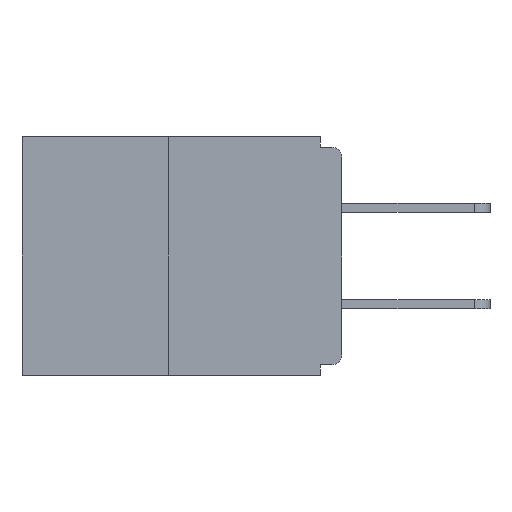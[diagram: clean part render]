
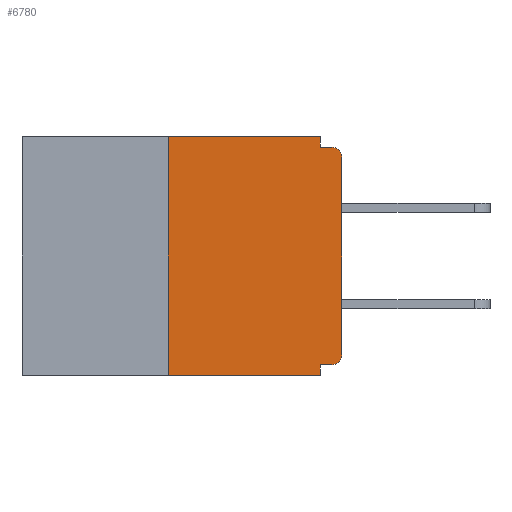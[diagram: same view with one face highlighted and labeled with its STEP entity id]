
A CAD part, left-side view. The second image highlights one B-rep face of the part: STEP entity #6780.
In plain terms, the highlighted planar face has unit normal (-1, 0, 0).
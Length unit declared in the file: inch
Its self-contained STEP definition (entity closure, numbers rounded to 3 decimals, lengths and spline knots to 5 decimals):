
#66 = CARTESIAN_POINT ( 'NONE',  ( 0., 0.031, 0. ) ) ;
#128 = CARTESIAN_POINT ( 'NONE',  ( 0., 0.015, -0.313 ) ) ;
#251 = CARTESIAN_POINT ( 'NONE',  ( 0., 0.031, -0.343 ) ) ;
#483 = DIRECTION ( 'NONE',  ( 1., 0., 0. ) ) ;
#576 = EDGE_CURVE ( 'NONE', #8437, #6505, #1379, .T. ) ;
#1377 = DIRECTION ( 'NONE',  ( 0., 0., -1. ) ) ;
#1379 = LINE ( 'NONE', #251, #6125 ) ;
#1640 = EDGE_CURVE ( 'NONE', #14112, #19363, #13053, .T. ) ;
#1816 = VERTEX_POINT ( 'NONE', #15189 ) ;
#2113 = LINE ( 'NONE', #4300, #10301 ) ;
#2531 = VECTOR ( 'NONE', #5734, 39.37008 ) ;
#2602 = FACE_OUTER_BOUND ( 'NONE', #16657, .T. ) ;
#3132 = EDGE_CURVE ( 'NONE', #1816, #14112, #12727, .T. ) ;
#3435 = CARTESIAN_POINT ( 'NONE',  ( 0., 0.031, 0. ) ) ;
#3496 = EDGE_CURVE ( 'NONE', #18222, #20248, #6762, .T. ) ;
#3988 = LINE ( 'NONE', #7442, #7696 ) ;
#4300 = CARTESIAN_POINT ( 'NONE',  ( 0., 0.46, -0.343 ) ) ;
#4327 = ORIENTED_EDGE ( 'NONE', *, *, #1640, .F. ) ;
#4531 = CARTESIAN_POINT ( 'NONE',  ( 0., 0.015, -0.015 ) ) ;
#4659 = DIRECTION ( 'NONE',  ( 0., 0., -1. ) ) ;
#5332 = CARTESIAN_POINT ( 'NONE',  ( 0., 0.031, -0.343 ) ) ;
#5734 = DIRECTION ( 'NONE',  ( 0., 0., 1. ) ) ;
#5997 = LINE ( 'NONE', #16172, #16929 ) ;
#6125 = VECTOR ( 'NONE', #15954, 39.37008 ) ;
#6214 = EDGE_CURVE ( 'NONE', #14409, #9686, #9053, .T. ) ;
#6505 = VERTEX_POINT ( 'NONE', #5332 ) ;
#6665 = CARTESIAN_POINT ( 'NONE',  ( 0., 0.46, 0. ) ) ;
#6762 = CIRCLE ( 'NONE', #8613, 0.015 ) ;
#6780 = ADVANCED_FACE ( 'NONE', ( #2602 ), #19461, .F. ) ;
#7053 = AXIS2_PLACEMENT_3D ( 'NONE', #6665, #483, #16252 ) ;
#7214 = EDGE_CURVE ( 'NONE', #12928, #6505, #2113, .T. ) ;
#7398 = DIRECTION ( 'NONE',  ( 0., 0., -1. ) ) ;
#7442 = CARTESIAN_POINT ( 'NONE',  ( 0., 0.25, 0. ) ) ;
#7696 = VECTOR ( 'NONE', #13715, 39.37008 ) ;
#8270 = DIRECTION ( 'NONE',  ( 0., 1., 0. ) ) ;
#8437 = VERTEX_POINT ( 'NONE', #9272 ) ;
#8613 = AXIS2_PLACEMENT_3D ( 'NONE', #9449, #10916, #1377 ) ;
#8761 = EDGE_CURVE ( 'NONE', #9686, #18222, #14700, .T. ) ;
#8899 = VECTOR ( 'NONE', #19779, 39.37008 ) ;
#9053 = CIRCLE ( 'NONE', #14910, 0.015 ) ;
#9259 = EDGE_CURVE ( 'NONE', #12928, #1816, #3988, .T. ) ;
#9272 = CARTESIAN_POINT ( 'NONE',  ( 0., 0.031, -0.328 ) ) ;
#9413 = ORIENTED_EDGE ( 'NONE', *, *, #8761, .T. ) ;
#9449 = CARTESIAN_POINT ( 'NONE',  ( 0., 0.015, -0.03 ) ) ;
#9601 = ORIENTED_EDGE ( 'NONE', *, *, #10444, .F. ) ;
#9686 = VERTEX_POINT ( 'NONE', #18036 ) ;
#10301 = VECTOR ( 'NONE', #10809, 39.37008 ) ;
#10444 = EDGE_CURVE ( 'NONE', #19363, #20248, #12618, .T. ) ;
#10809 = DIRECTION ( 'NONE',  ( 0., -1., 0. ) ) ;
#10916 = DIRECTION ( 'NONE',  ( -1., 0., 0. ) ) ;
#11150 = CARTESIAN_POINT ( 'NONE',  ( 0., 0.46, 0. ) ) ;
#11790 = ORIENTED_EDGE ( 'NONE', *, *, #19508, .F. ) ;
#12618 = LINE ( 'NONE', #18275, #8899 ) ;
#12727 = LINE ( 'NONE', #11150, #13249 ) ;
#12928 = VERTEX_POINT ( 'NONE', #14136 ) ;
#13053 = LINE ( 'NONE', #66, #14061 ) ;
#13249 = VECTOR ( 'NONE', #19274, 39.37008 ) ;
#13715 = DIRECTION ( 'NONE',  ( 0., 0., 1. ) ) ;
#14061 = VECTOR ( 'NONE', #4659, 39.37008 ) ;
#14112 = VERTEX_POINT ( 'NONE', #3435 ) ;
#14136 = CARTESIAN_POINT ( 'NONE',  ( 0., 0.25, -0.343 ) ) ;
#14409 = VERTEX_POINT ( 'NONE', #18959 ) ;
#14455 = DIRECTION ( 'NONE',  ( -1., 0., 0. ) ) ;
#14700 = LINE ( 'NONE', #15370, #2531 ) ;
#14910 = AXIS2_PLACEMENT_3D ( 'NONE', #128, #14455, #7398 ) ;
#15189 = CARTESIAN_POINT ( 'NONE',  ( 0., 0.25, 0. ) ) ;
#15370 = CARTESIAN_POINT ( 'NONE',  ( 0., 0., 0. ) ) ;
#15902 = CARTESIAN_POINT ( 'NONE',  ( 0., 0., -0.03 ) ) ;
#15954 = DIRECTION ( 'NONE',  ( 0., 0., -1. ) ) ;
#16172 = CARTESIAN_POINT ( 'NONE',  ( 0., 0., -0.328 ) ) ;
#16252 = DIRECTION ( 'NONE',  ( 0., 0., -1. ) ) ;
#16657 = EDGE_LOOP ( 'NONE', ( #17831, #20264, #17310, #20112, #11790, #16899, #9413, #17422, #9601, #4327 ) ) ;
#16899 = ORIENTED_EDGE ( 'NONE', *, *, #6214, .T. ) ;
#16929 = VECTOR ( 'NONE', #8270, 39.37008 ) ;
#17310 = ORIENTED_EDGE ( 'NONE', *, *, #7214, .T. ) ;
#17422 = ORIENTED_EDGE ( 'NONE', *, *, #3496, .T. ) ;
#17831 = ORIENTED_EDGE ( 'NONE', *, *, #3132, .F. ) ;
#18036 = CARTESIAN_POINT ( 'NONE',  ( 0., 0., -0.313 ) ) ;
#18222 = VERTEX_POINT ( 'NONE', #15902 ) ;
#18275 = CARTESIAN_POINT ( 'NONE',  ( 0., 0., -0.015 ) ) ;
#18764 = CARTESIAN_POINT ( 'NONE',  ( 0., 0.031, -0.015 ) ) ;
#18959 = CARTESIAN_POINT ( 'NONE',  ( 0., 0.015, -0.328 ) ) ;
#19274 = DIRECTION ( 'NONE',  ( 0., -1., 0. ) ) ;
#19363 = VERTEX_POINT ( 'NONE', #18764 ) ;
#19461 = PLANE ( 'NONE',  #7053 ) ;
#19508 = EDGE_CURVE ( 'NONE', #14409, #8437, #5997, .T. ) ;
#19779 = DIRECTION ( 'NONE',  ( 0., -1., 0. ) ) ;
#20112 = ORIENTED_EDGE ( 'NONE', *, *, #576, .F. ) ;
#20248 = VERTEX_POINT ( 'NONE', #4531 ) ;
#20264 = ORIENTED_EDGE ( 'NONE', *, *, #9259, .F. ) ;
